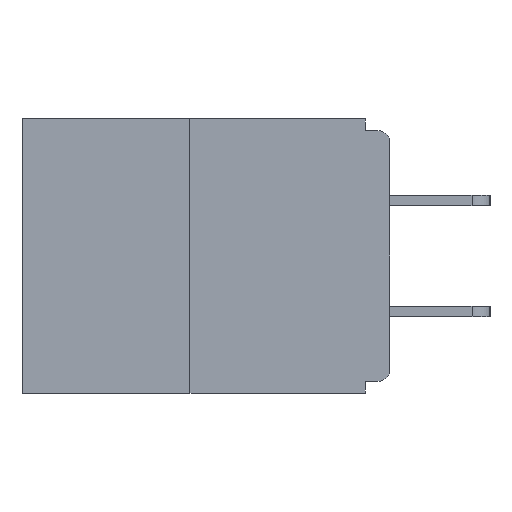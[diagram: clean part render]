
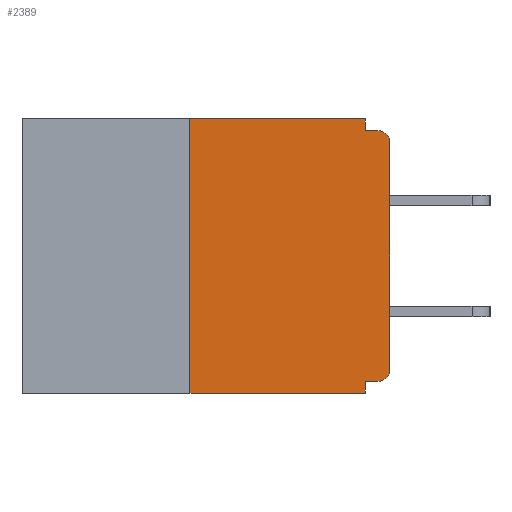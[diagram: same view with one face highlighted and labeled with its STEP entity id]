
A CAD part, left-side view. The second image highlights one B-rep face of the part: STEP entity #2389.
In plain terms, the highlighted planar face has unit normal (-1, 0, 0).
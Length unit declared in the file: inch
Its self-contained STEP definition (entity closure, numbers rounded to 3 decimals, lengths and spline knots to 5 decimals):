
#305 = DIRECTION ( 'NONE',  ( 0., 0., -1. ) ) ;
#312 = DIRECTION ( 'NONE',  ( -1., 0., 0. ) ) ;
#925 = CARTESIAN_POINT ( 'NONE',  ( 0., 0.46, 0. ) ) ;
#1047 = CARTESIAN_POINT ( 'NONE',  ( 0., 0.25, 0. ) ) ;
#2305 = VERTEX_POINT ( 'NONE', #2886 ) ;
#2389 = ADVANCED_FACE ( 'NONE', ( #3005 ), #8100, .F. ) ;
#2430 = ORIENTED_EDGE ( 'NONE', *, *, #28997, .T. ) ;
#2454 = ORIENTED_EDGE ( 'NONE', *, *, #14483, .F. ) ;
#2886 = CARTESIAN_POINT ( 'NONE',  ( 0., 0.25, 0. ) ) ;
#3005 = FACE_OUTER_BOUND ( 'NONE', #17770, .T. ) ;
#3392 = DIRECTION ( 'NONE',  ( 1., 0., 0. ) ) ;
#4009 = CARTESIAN_POINT ( 'NONE',  ( 0., 0., -0.03 ) ) ;
#4462 = CARTESIAN_POINT ( 'NONE',  ( 0., 0.015, -0.015 ) ) ;
#4470 = LINE ( 'NONE', #11610, #27561 ) ;
#5257 = LINE ( 'NONE', #20328, #8561 ) ;
#5738 = CARTESIAN_POINT ( 'NONE',  ( 0., 0.031, 0. ) ) ;
#5800 = VERTEX_POINT ( 'NONE', #4009 ) ;
#5820 = AXIS2_PLACEMENT_3D ( 'NONE', #925, #3392, #12522 ) ;
#5867 = EDGE_CURVE ( 'NONE', #25439, #8593, #5257, .T. ) ;
#7801 = ORIENTED_EDGE ( 'NONE', *, *, #19169, .F. ) ;
#8100 = PLANE ( 'NONE',  #5820 ) ;
#8561 = VECTOR ( 'NONE', #13336, 39.37008 ) ;
#8593 = VERTEX_POINT ( 'NONE', #24502 ) ;
#8866 = EDGE_CURVE ( 'NONE', #26995, #17816, #12073, .T. ) ;
#9247 = ORIENTED_EDGE ( 'NONE', *, *, #21747, .F. ) ;
#9617 = CARTESIAN_POINT ( 'NONE',  ( 0., 0.015, -0.313 ) ) ;
#10099 = CARTESIAN_POINT ( 'NONE',  ( 0., 0., -0.313 ) ) ;
#10205 = CARTESIAN_POINT ( 'NONE',  ( 0., 0.46, -0.343 ) ) ;
#10347 = VECTOR ( 'NONE', #24543, 39.37008 ) ;
#10488 = CIRCLE ( 'NONE', #27545, 0.015 ) ;
#11161 = CARTESIAN_POINT ( 'NONE',  ( 0., 0.031, -0.343 ) ) ;
#11387 = CARTESIAN_POINT ( 'NONE',  ( 0., 0.015, -0.03 ) ) ;
#11610 = CARTESIAN_POINT ( 'NONE',  ( 0., 0., -0.015 ) ) ;
#12073 = LINE ( 'NONE', #10205, #22352 ) ;
#12109 = CARTESIAN_POINT ( 'NONE',  ( 0., 0.031, 0. ) ) ;
#12413 = CARTESIAN_POINT ( 'NONE',  ( 0., 0.031, -0.015 ) ) ;
#12522 = DIRECTION ( 'NONE',  ( 0., 0., -1. ) ) ;
#13220 = EDGE_CURVE ( 'NONE', #25375, #5800, #24713, .T. ) ;
#13237 = VERTEX_POINT ( 'NONE', #4462 ) ;
#13323 = LINE ( 'NONE', #28084, #18111 ) ;
#13336 = DIRECTION ( 'NONE',  ( 0., 1., 0. ) ) ;
#14483 = EDGE_CURVE ( 'NONE', #2305, #28681, #16256, .T. ) ;
#15111 = EDGE_CURVE ( 'NONE', #26995, #2305, #24309, .T. ) ;
#16206 = DIRECTION ( 'NONE',  ( 0., -1., 0. ) ) ;
#16256 = LINE ( 'NONE', #22023, #26179 ) ;
#16606 = ORIENTED_EDGE ( 'NONE', *, *, #13220, .T. ) ;
#16703 = DIRECTION ( 'NONE',  ( 0., 0., -1. ) ) ;
#17347 = VECTOR ( 'NONE', #30003, 39.37008 ) ;
#17501 = DIRECTION ( 'NONE',  ( 0., -1., 0. ) ) ;
#17511 = VERTEX_POINT ( 'NONE', #12413 ) ;
#17770 = EDGE_LOOP ( 'NONE', ( #2454, #29760, #26808, #23398, #29881, #2430, #16606, #27752, #7801, #9247 ) ) ;
#17816 = VERTEX_POINT ( 'NONE', #11161 ) ;
#18010 = AXIS2_PLACEMENT_3D ( 'NONE', #11387, #20912, #18857 ) ;
#18111 = VECTOR ( 'NONE', #23837, 39.37008 ) ;
#18271 = VECTOR ( 'NONE', #305, 39.37008 ) ;
#18857 = DIRECTION ( 'NONE',  ( 0., 0., -1. ) ) ;
#19169 = EDGE_CURVE ( 'NONE', #17511, #13237, #4470, .T. ) ;
#19384 = CIRCLE ( 'NONE', #18010, 0.015 ) ;
#20328 = CARTESIAN_POINT ( 'NONE',  ( 0., 0., -0.328 ) ) ;
#20912 = DIRECTION ( 'NONE',  ( -1., 0., 0. ) ) ;
#21570 = EDGE_CURVE ( 'NONE', #5800, #13237, #19384, .T. ) ;
#21700 = DIRECTION ( 'NONE',  ( 0., -1., 0. ) ) ;
#21747 = EDGE_CURVE ( 'NONE', #28681, #17511, #29263, .T. ) ;
#22023 = CARTESIAN_POINT ( 'NONE',  ( 0., 0.46, 0. ) ) ;
#22352 = VECTOR ( 'NONE', #21700, 39.37008 ) ;
#23398 = ORIENTED_EDGE ( 'NONE', *, *, #30254, .F. ) ;
#23837 = DIRECTION ( 'NONE',  ( 0., 0., -1. ) ) ;
#24309 = LINE ( 'NONE', #1047, #10347 ) ;
#24502 = CARTESIAN_POINT ( 'NONE',  ( 0., 0.031, -0.328 ) ) ;
#24543 = DIRECTION ( 'NONE',  ( 0., 0., 1. ) ) ;
#24713 = LINE ( 'NONE', #30204, #17347 ) ;
#25375 = VERTEX_POINT ( 'NONE', #10099 ) ;
#25439 = VERTEX_POINT ( 'NONE', #26314 ) ;
#26179 = VECTOR ( 'NONE', #17501, 39.37008 ) ;
#26314 = CARTESIAN_POINT ( 'NONE',  ( 0., 0.015, -0.328 ) ) ;
#26808 = ORIENTED_EDGE ( 'NONE', *, *, #8866, .T. ) ;
#26995 = VERTEX_POINT ( 'NONE', #29113 ) ;
#27545 = AXIS2_PLACEMENT_3D ( 'NONE', #9617, #312, #16703 ) ;
#27561 = VECTOR ( 'NONE', #16206, 39.37008 ) ;
#27752 = ORIENTED_EDGE ( 'NONE', *, *, #21570, .T. ) ;
#28084 = CARTESIAN_POINT ( 'NONE',  ( 0., 0.031, -0.343 ) ) ;
#28681 = VERTEX_POINT ( 'NONE', #5738 ) ;
#28997 = EDGE_CURVE ( 'NONE', #25439, #25375, #10488, .T. ) ;
#29113 = CARTESIAN_POINT ( 'NONE',  ( 0., 0.25, -0.343 ) ) ;
#29263 = LINE ( 'NONE', #12109, #18271 ) ;
#29760 = ORIENTED_EDGE ( 'NONE', *, *, #15111, .F. ) ;
#29881 = ORIENTED_EDGE ( 'NONE', *, *, #5867, .F. ) ;
#30003 = DIRECTION ( 'NONE',  ( 0., 0., 1. ) ) ;
#30204 = CARTESIAN_POINT ( 'NONE',  ( 0., 0., 0. ) ) ;
#30254 = EDGE_CURVE ( 'NONE', #8593, #17816, #13323, .T. ) ;
